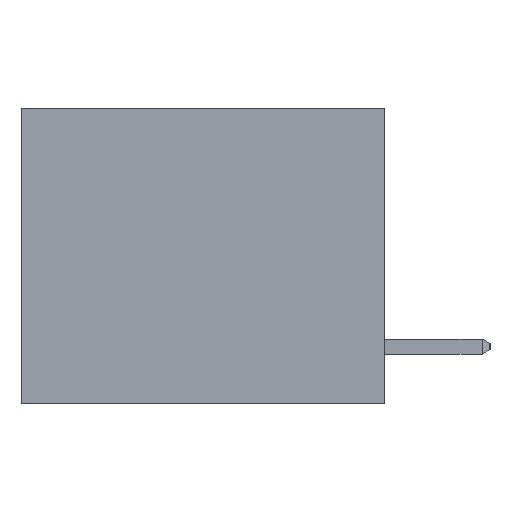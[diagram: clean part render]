
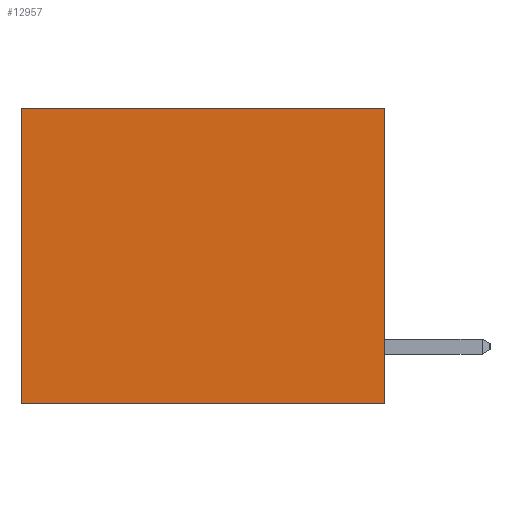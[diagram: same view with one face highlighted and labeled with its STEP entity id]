
A CAD part, left-side view. The second image highlights one B-rep face of the part: STEP entity #12957.
In plain terms, the highlighted planar face has unit normal (-1, 0, 0).
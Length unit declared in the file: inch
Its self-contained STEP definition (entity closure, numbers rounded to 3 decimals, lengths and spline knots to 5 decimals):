
#225 = CARTESIAN_POINT ( 'NONE',  ( 0.3165, 0., -0.49 ) ) ;
#448 = CARTESIAN_POINT ( 'NONE',  ( 0.3165, 0.6, -0.49 ) ) ;
#530 = LINE ( 'NONE', #18397, #16976 ) ;
#647 = DIRECTION ( 'NONE',  ( 0., 0., -1. ) ) ;
#1110 = EDGE_CURVE ( 'NONE', #3236, #13885, #17995, .T. ) ;
#1585 = CARTESIAN_POINT ( 'NONE',  ( 0.3165, 0.6, 0. ) ) ;
#1684 = ORIENTED_EDGE ( 'NONE', *, *, #1110, .T. ) ;
#1841 = DIRECTION ( 'NONE',  ( 0., 1., 0. ) ) ;
#1875 = EDGE_CURVE ( 'NONE', #17630, #4774, #8751, .T. ) ;
#2418 = VECTOR ( 'NONE', #1841, 39.37008 ) ;
#3236 = VERTEX_POINT ( 'NONE', #1585 ) ;
#4774 = VERTEX_POINT ( 'NONE', #6057 ) ;
#5523 = VECTOR ( 'NONE', #647, 39.37008 ) ;
#6057 = CARTESIAN_POINT ( 'NONE',  ( 0.3165, 0., -0.49 ) ) ;
#6383 = CARTESIAN_POINT ( 'NONE',  ( 0.3165, 0., 0. ) ) ;
#6919 = LINE ( 'NONE', #225, #2418 ) ;
#7001 = ORIENTED_EDGE ( 'NONE', *, *, #16575, .T. ) ;
#7313 = EDGE_LOOP ( 'NONE', ( #1684, #13433, #13413, #7001 ) ) ;
#8751 = LINE ( 'NONE', #10931, #12523 ) ;
#8867 = PLANE ( 'NONE',  #20085 ) ;
#9371 = DIRECTION ( 'NONE',  ( 0., 0., -1. ) ) ;
#10931 = CARTESIAN_POINT ( 'NONE',  ( 0.3165, 0., -0.49 ) ) ;
#11745 = CARTESIAN_POINT ( 'NONE',  ( 0.3165, 0.6, -0.49 ) ) ;
#11976 = DIRECTION ( 'NONE',  ( 1., 0., 0. ) ) ;
#12014 = DIRECTION ( 'NONE',  ( 0., 1., 0. ) ) ;
#12523 = VECTOR ( 'NONE', #9371, 39.37008 ) ;
#12957 = ADVANCED_FACE ( 'NONE', ( #14187 ), #8867, .F. ) ;
#13202 = EDGE_CURVE ( 'NONE', #4774, #13885, #6919, .T. ) ;
#13413 = ORIENTED_EDGE ( 'NONE', *, *, #1875, .F. ) ;
#13433 = ORIENTED_EDGE ( 'NONE', *, *, #13202, .F. ) ;
#13885 = VERTEX_POINT ( 'NONE', #11745 ) ;
#14187 = FACE_OUTER_BOUND ( 'NONE', #7313, .T. ) ;
#16575 = EDGE_CURVE ( 'NONE', #17630, #3236, #530, .T. ) ;
#16744 = CARTESIAN_POINT ( 'NONE',  ( 0.3165, 0., -0.49 ) ) ;
#16976 = VECTOR ( 'NONE', #12014, 39.37008 ) ;
#17630 = VERTEX_POINT ( 'NONE', #6383 ) ;
#17995 = LINE ( 'NONE', #448, #5523 ) ;
#18397 = CARTESIAN_POINT ( 'NONE',  ( 0.3165, 0., 0. ) ) ;
#18496 = DIRECTION ( 'NONE',  ( 0., 0., -1. ) ) ;
#20085 = AXIS2_PLACEMENT_3D ( 'NONE', #16744, #11976, #18496 ) ;
